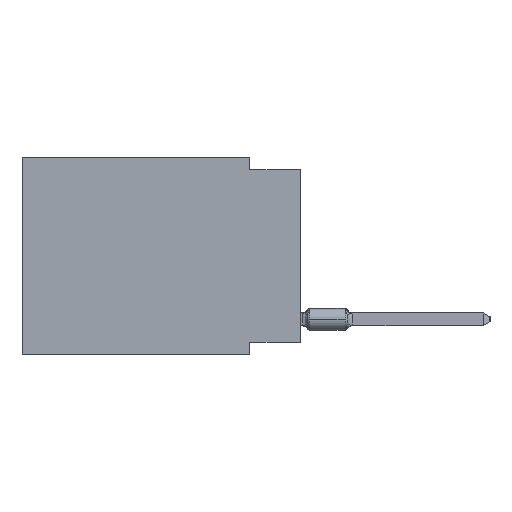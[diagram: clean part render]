
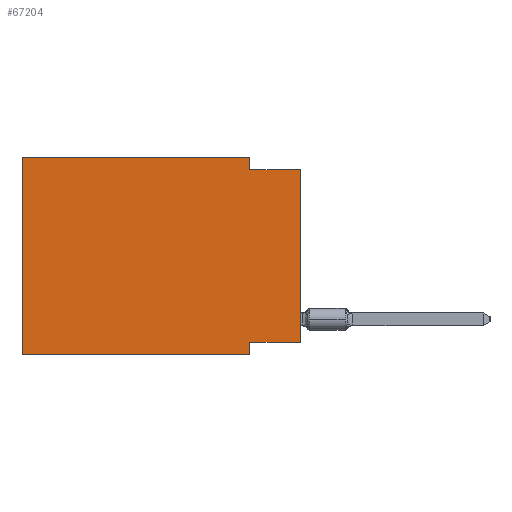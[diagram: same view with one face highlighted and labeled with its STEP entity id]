
A CAD part, left-side view. The second image highlights one B-rep face of the part: STEP entity #67204.
In plain terms, the highlighted planar face has unit normal (-1, 0, 0).
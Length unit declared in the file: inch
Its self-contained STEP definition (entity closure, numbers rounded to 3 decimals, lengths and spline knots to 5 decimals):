
#2669 = DIRECTION ( 'NONE',  ( 0., -1., 0. ) ) ;
#5375 = EDGE_CURVE ( 'NONE', #75829, #48436, #72304, .T. ) ;
#5440 = EDGE_LOOP ( 'NONE', ( #74208, #71782, #63463, #66790, #14620, #9598, #31984, #27545 ) ) ;
#6753 = EDGE_CURVE ( 'NONE', #75829, #47620, #44821, .T. ) ;
#7034 = VECTOR ( 'NONE', #46479, 39.37008 ) ;
#9598 = ORIENTED_EDGE ( 'NONE', *, *, #56373, .T. ) ;
#10040 = CARTESIAN_POINT ( 'NONE',  ( 0., 0., -0.365 ) ) ;
#14620 = ORIENTED_EDGE ( 'NONE', *, *, #66482, .F. ) ;
#14621 = VERTEX_POINT ( 'NONE', #55378 ) ;
#14664 = EDGE_CURVE ( 'NONE', #57329, #48436, #62750, .T. ) ;
#16998 = CARTESIAN_POINT ( 'NONE',  ( 0., 0.55, 0. ) ) ;
#18811 = CARTESIAN_POINT ( 'NONE',  ( 0., 0., 0. ) ) ;
#20708 = CARTESIAN_POINT ( 'NONE',  ( 0., 0., -0.365 ) ) ;
#22650 = LINE ( 'NONE', #68857, #7034 ) ;
#23776 = VERTEX_POINT ( 'NONE', #63525 ) ;
#25106 = LINE ( 'NONE', #16998, #66378 ) ;
#27026 = VECTOR ( 'NONE', #2669, 39.37008 ) ;
#27545 = ORIENTED_EDGE ( 'NONE', *, *, #6753, .F. ) ;
#28110 = FACE_OUTER_BOUND ( 'NONE', #5440, .T. ) ;
#28679 = DIRECTION ( 'NONE',  ( 0., 0., 1. ) ) ;
#29454 = LINE ( 'NONE', #34920, #71473 ) ;
#30133 = VECTOR ( 'NONE', #65672, 39.37008 ) ;
#31984 = ORIENTED_EDGE ( 'NONE', *, *, #50516, .F. ) ;
#32151 = DIRECTION ( 'NONE',  ( 0., 0., -1. ) ) ;
#32613 = VECTOR ( 'NONE', #32151, 39.37008 ) ;
#33292 = CARTESIAN_POINT ( 'NONE',  ( 0., 0.1, 0. ) ) ;
#34350 = PLANE ( 'NONE',  #57817 ) ;
#34920 = CARTESIAN_POINT ( 'NONE',  ( 0., 0.55, 0. ) ) ;
#35045 = CARTESIAN_POINT ( 'NONE',  ( 0., 0.1, -0.025 ) ) ;
#40837 = DIRECTION ( 'NONE',  ( 0., -1., 0. ) ) ;
#43160 = VECTOR ( 'NONE', #43230, 39.37008 ) ;
#43230 = DIRECTION ( 'NONE',  ( 0., -1., 0. ) ) ;
#43466 = LINE ( 'NONE', #33292, #32613 ) ;
#43611 = LINE ( 'NONE', #72880, #43160 ) ;
#43904 = CARTESIAN_POINT ( 'NONE',  ( 0., 0.1, -0.39 ) ) ;
#44359 = EDGE_CURVE ( 'NONE', #23776, #63599, #25106, .T. ) ;
#44821 = LINE ( 'NONE', #10040, #57064 ) ;
#46479 = DIRECTION ( 'NONE',  ( 0., 0., -1. ) ) ;
#46827 = DIRECTION ( 'NONE',  ( 0., 0., -1. ) ) ;
#47620 = VERTEX_POINT ( 'NONE', #51400 ) ;
#48436 = VERTEX_POINT ( 'NONE', #64399 ) ;
#50516 = EDGE_CURVE ( 'NONE', #47620, #54988, #22650, .T. ) ;
#51400 = CARTESIAN_POINT ( 'NONE',  ( 0., 0.1, -0.365 ) ) ;
#54988 = VERTEX_POINT ( 'NONE', #43904 ) ;
#55378 = CARTESIAN_POINT ( 'NONE',  ( 0., 0.55, -0.39 ) ) ;
#56141 = CARTESIAN_POINT ( 'NONE',  ( 0., 0., -0.025 ) ) ;
#56373 = EDGE_CURVE ( 'NONE', #14621, #54988, #43611, .T. ) ;
#57064 = VECTOR ( 'NONE', #57290, 39.37008 ) ;
#57290 = DIRECTION ( 'NONE',  ( 0., 1., 0. ) ) ;
#57329 = VERTEX_POINT ( 'NONE', #35045 ) ;
#57402 = CARTESIAN_POINT ( 'NONE',  ( 0., 0.55, 0. ) ) ;
#57817 = AXIS2_PLACEMENT_3D ( 'NONE', #57402, #69483, #46827 ) ;
#62750 = LINE ( 'NONE', #56141, #27026 ) ;
#63463 = ORIENTED_EDGE ( 'NONE', *, *, #64428, .F. ) ;
#63525 = CARTESIAN_POINT ( 'NONE',  ( 0., 0.55, 0. ) ) ;
#63599 = VERTEX_POINT ( 'NONE', #69686 ) ;
#64399 = CARTESIAN_POINT ( 'NONE',  ( 0., 0., -0.025 ) ) ;
#64428 = EDGE_CURVE ( 'NONE', #63599, #57329, #43466, .T. ) ;
#65672 = DIRECTION ( 'NONE',  ( 0., 0., 1. ) ) ;
#66378 = VECTOR ( 'NONE', #40837, 39.37008 ) ;
#66482 = EDGE_CURVE ( 'NONE', #14621, #23776, #29454, .T. ) ;
#66790 = ORIENTED_EDGE ( 'NONE', *, *, #44359, .F. ) ;
#67204 = ADVANCED_FACE ( 'NONE', ( #28110 ), #34350, .F. ) ;
#68857 = CARTESIAN_POINT ( 'NONE',  ( 0., 0.1, -0.39 ) ) ;
#69483 = DIRECTION ( 'NONE',  ( 1., 0., 0. ) ) ;
#69686 = CARTESIAN_POINT ( 'NONE',  ( 0., 0.1, 0. ) ) ;
#71473 = VECTOR ( 'NONE', #28679, 39.37008 ) ;
#71782 = ORIENTED_EDGE ( 'NONE', *, *, #14664, .F. ) ;
#72304 = LINE ( 'NONE', #18811, #30133 ) ;
#72880 = CARTESIAN_POINT ( 'NONE',  ( 0., 0.55, -0.39 ) ) ;
#74208 = ORIENTED_EDGE ( 'NONE', *, *, #5375, .T. ) ;
#75829 = VERTEX_POINT ( 'NONE', #20708 ) ;
